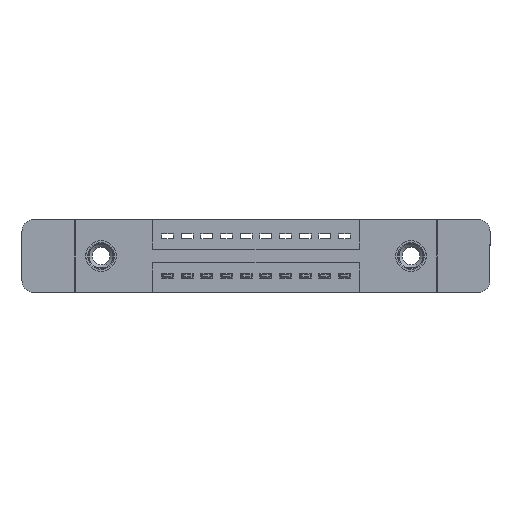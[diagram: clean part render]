
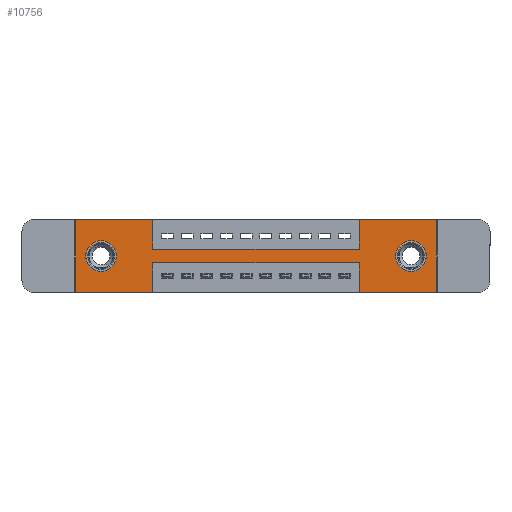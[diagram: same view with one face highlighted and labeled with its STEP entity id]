
A CAD part, front view. The second image highlights one B-rep face of the part: STEP entity #10756.
In plain terms, the highlighted planar face has unit normal (0, -1, 0).
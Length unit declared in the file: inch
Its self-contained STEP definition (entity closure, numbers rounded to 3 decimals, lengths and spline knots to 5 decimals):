
#69 = CARTESIAN_POINT ( 'NONE',  ( 0.3925, 0., -0.37 ) ) ;
#352 = VECTOR ( 'NONE', #3452, 39.37008 ) ;
#764 = VECTOR ( 'NONE', #14579, 39.37008 ) ;
#906 = LINE ( 'NONE', #8370, #14106 ) ;
#907 = ORIENTED_EDGE ( 'NONE', *, *, #7515, .T. ) ;
#1094 = DIRECTION ( 'NONE',  ( 1., 0., 0. ) ) ;
#1175 = VECTOR ( 'NONE', #15519, 39.37008 ) ;
#1199 = CARTESIAN_POINT ( 'NONE',  ( 0., 0., -0.37 ) ) ;
#1305 = DIRECTION ( 'NONE',  ( 1., 0., 0. ) ) ;
#1678 = DIRECTION ( 'NONE',  ( 0., 0., 1. ) ) ;
#1769 = LINE ( 'NONE', #69, #16605 ) ;
#1973 = EDGE_CURVE ( 'NONE', #7107, #16016, #13414, .T. ) ;
#2114 = FACE_OUTER_BOUND ( 'NONE', #6255, .T. ) ;
#2141 = VERTEX_POINT ( 'NONE', #15989 ) ;
#2217 = LINE ( 'NONE', #6424, #5238 ) ;
#2262 = ORIENTED_EDGE ( 'NONE', *, *, #8040, .F. ) ;
#2483 = DIRECTION ( 'NONE',  ( 0., -1., 0. ) ) ;
#2630 = VECTOR ( 'NONE', #10622, 39.37008 ) ;
#2729 = EDGE_CURVE ( 'NONE', #5162, #9375, #3029, .T. ) ;
#2741 = ORIENTED_EDGE ( 'NONE', *, *, #2940, .F. ) ;
#2897 = ORIENTED_EDGE ( 'NONE', *, *, #10849, .F. ) ;
#2940 = EDGE_CURVE ( 'NONE', #7504, #8922, #15925, .T. ) ;
#3029 = LINE ( 'NONE', #4997, #14016 ) ;
#3164 = CIRCLE ( 'NONE', #3179, 0.078 ) ;
#3179 = AXIS2_PLACEMENT_3D ( 'NONE', #3702, #4996, #6303 ) ;
#3452 = DIRECTION ( 'NONE',  ( -1., 0., 0. ) ) ;
#3506 = AXIS2_PLACEMENT_3D ( 'NONE', #15658, #6880, #13429 ) ;
#3511 = ORIENTED_EDGE ( 'NONE', *, *, #2729, .F. ) ;
#3568 = CARTESIAN_POINT ( 'NONE',  ( 1.4425, 0., 0. ) ) ;
#3702 = CARTESIAN_POINT ( 'NONE',  ( 1.705, 0., -0.185 ) ) ;
#3822 = DIRECTION ( 'NONE',  ( 1., 0., 0. ) ) ;
#3981 = CARTESIAN_POINT ( 'NONE',  ( 1.4425, 0., -0.22 ) ) ;
#4023 = CIRCLE ( 'NONE', #3506, 0.078 ) ;
#4073 = ORIENTED_EDGE ( 'NONE', *, *, #15768, .F. ) ;
#4182 = CARTESIAN_POINT ( 'NONE',  ( 0.3925, 0., 0. ) ) ;
#4228 = CARTESIAN_POINT ( 'NONE',  ( 0.13, 0., -0.107 ) ) ;
#4996 = DIRECTION ( 'NONE',  ( 0., 1., 0. ) ) ;
#4997 = CARTESIAN_POINT ( 'NONE',  ( 1.4425, 0., 0. ) ) ;
#5162 = VERTEX_POINT ( 'NONE', #7368 ) ;
#5234 = VERTEX_POINT ( 'NONE', #11166 ) ;
#5238 = VECTOR ( 'NONE', #11711, 39.37008 ) ;
#5241 = PLANE ( 'NONE',  #15727 ) ;
#5433 = VERTEX_POINT ( 'NONE', #11720 ) ;
#5545 = FACE_BOUND ( 'NONE', #5600, .T. ) ;
#5600 = EDGE_LOOP ( 'NONE', ( #14666, #7173 ) ) ;
#5824 = AXIS2_PLACEMENT_3D ( 'NONE', #11332, #7590, #7358 ) ;
#6061 = CIRCLE ( 'NONE', #14182, 0.078 ) ;
#6255 = EDGE_LOOP ( 'NONE', ( #2262, #4073, #2897, #14970, #8181, #15022, #3511, #14803, #2741, #13793, #12259, #10843 ) ) ;
#6303 = DIRECTION ( 'NONE',  ( 0., 0., -1. ) ) ;
#6424 = CARTESIAN_POINT ( 'NONE',  ( 0., 0., -0.37 ) ) ;
#6515 = CARTESIAN_POINT ( 'NONE',  ( 0.13, 0., -0.263 ) ) ;
#6685 = LINE ( 'NONE', #11953, #2630 ) ;
#6837 = EDGE_CURVE ( 'NONE', #2141, #7504, #12170, .T. ) ;
#6880 = DIRECTION ( 'NONE',  ( 0., 1., 0. ) ) ;
#6883 = DIRECTION ( 'NONE',  ( 0., 0., -1. ) ) ;
#6906 = EDGE_CURVE ( 'NONE', #7212, #5433, #2217, .T. ) ;
#7019 = LINE ( 'NONE', #11229, #352 ) ;
#7107 = VERTEX_POINT ( 'NONE', #11995 ) ;
#7173 = ORIENTED_EDGE ( 'NONE', *, *, #1973, .T. ) ;
#7212 = VERTEX_POINT ( 'NONE', #14894 ) ;
#7358 = DIRECTION ( 'NONE',  ( 0., 0., -1. ) ) ;
#7368 = CARTESIAN_POINT ( 'NONE',  ( 1.4425, 0., -0.15 ) ) ;
#7500 = ORIENTED_EDGE ( 'NONE', *, *, #12958, .T. ) ;
#7504 = VERTEX_POINT ( 'NONE', #12983 ) ;
#7515 = EDGE_CURVE ( 'NONE', #12425, #14979, #4023, .T. ) ;
#7590 = DIRECTION ( 'NONE',  ( 0., 1., 0. ) ) ;
#7779 = CARTESIAN_POINT ( 'NONE',  ( 1.4425, 0., -0.37 ) ) ;
#8040 = EDGE_CURVE ( 'NONE', #11811, #7212, #1769, .T. ) ;
#8067 = LINE ( 'NONE', #15754, #764 ) ;
#8181 = ORIENTED_EDGE ( 'NONE', *, *, #15499, .F. ) ;
#8287 = EDGE_CURVE ( 'NONE', #16415, #16197, #7019, .T. ) ;
#8370 = CARTESIAN_POINT ( 'NONE',  ( 1.4425, 0., -0.37 ) ) ;
#8707 = DIRECTION ( 'NONE',  ( 0., 0., 1. ) ) ;
#8922 = VERTEX_POINT ( 'NONE', #13014 ) ;
#9056 = VERTEX_POINT ( 'NONE', #3981 ) ;
#9169 = CARTESIAN_POINT ( 'NONE',  ( 0., 0., 0. ) ) ;
#9335 = DIRECTION ( 'NONE',  ( 0., 0., -1. ) ) ;
#9375 = VERTEX_POINT ( 'NONE', #3568 ) ;
#10256 = EDGE_LOOP ( 'NONE', ( #7500, #907 ) ) ;
#10622 = DIRECTION ( 'NONE',  ( 0., 0., 1. ) ) ;
#10756 = ADVANCED_FACE ( 'NONE', ( #5545, #11655, #2114 ), #5241, .T. ) ;
#10843 = ORIENTED_EDGE ( 'NONE', *, *, #6906, .F. ) ;
#10849 = EDGE_CURVE ( 'NONE', #16197, #9056, #906, .T. ) ;
#11002 = CARTESIAN_POINT ( 'NONE',  ( 1.705, 0., -0.107 ) ) ;
#11166 = CARTESIAN_POINT ( 'NONE',  ( 1.835, 0., 0. ) ) ;
#11229 = CARTESIAN_POINT ( 'NONE',  ( 0., 0., -0.37 ) ) ;
#11332 = CARTESIAN_POINT ( 'NONE',  ( 1.705, 0., -0.185 ) ) ;
#11397 = DIRECTION ( 'NONE',  ( 0., 1., 0. ) ) ;
#11622 = DIRECTION ( 'NONE',  ( 0., 0., 1. ) ) ;
#11655 = FACE_BOUND ( 'NONE', #10256, .T. ) ;
#11711 = DIRECTION ( 'NONE',  ( -1., 0., 0. ) ) ;
#11720 = CARTESIAN_POINT ( 'NONE',  ( 0., 0., -0.37 ) ) ;
#11811 = VERTEX_POINT ( 'NONE', #14137 ) ;
#11905 = VECTOR ( 'NONE', #1094, 39.37008 ) ;
#11953 = CARTESIAN_POINT ( 'NONE',  ( 0., 0., 0. ) ) ;
#11961 = CARTESIAN_POINT ( 'NONE',  ( 1.835, 0., -0.37 ) ) ;
#11995 = CARTESIAN_POINT ( 'NONE',  ( 1.705, 0., -0.263 ) ) ;
#12170 = LINE ( 'NONE', #14125, #14434 ) ;
#12259 = ORIENTED_EDGE ( 'NONE', *, *, #13176, .F. ) ;
#12425 = VERTEX_POINT ( 'NONE', #6515 ) ;
#12474 = VECTOR ( 'NONE', #6883, 39.37008 ) ;
#12883 = DIRECTION ( 'NONE',  ( 0., 0., -1. ) ) ;
#12958 = EDGE_CURVE ( 'NONE', #14979, #12425, #6061, .T. ) ;
#12983 = CARTESIAN_POINT ( 'NONE',  ( 0.3925, 0., 0. ) ) ;
#13014 = CARTESIAN_POINT ( 'NONE',  ( 0.3925, 0., -0.15 ) ) ;
#13176 = EDGE_CURVE ( 'NONE', #5433, #2141, #6685, .T. ) ;
#13414 = CIRCLE ( 'NONE', #5824, 0.078 ) ;
#13429 = DIRECTION ( 'NONE',  ( 0., 0., 1. ) ) ;
#13745 = LINE ( 'NONE', #9169, #16186 ) ;
#13793 = ORIENTED_EDGE ( 'NONE', *, *, #6837, .F. ) ;
#13996 = CARTESIAN_POINT ( 'NONE',  ( 0.3925, 0., -0.22 ) ) ;
#14016 = VECTOR ( 'NONE', #8707, 39.37008 ) ;
#14106 = VECTOR ( 'NONE', #1678, 39.37008 ) ;
#14125 = CARTESIAN_POINT ( 'NONE',  ( 0., 0., 0. ) ) ;
#14137 = CARTESIAN_POINT ( 'NONE',  ( 0.3925, 0., -0.22 ) ) ;
#14182 = AXIS2_PLACEMENT_3D ( 'NONE', #15486, #11397, #11622 ) ;
#14434 = VECTOR ( 'NONE', #3822, 39.37008 ) ;
#14579 = DIRECTION ( 'NONE',  ( 0., 0., -1. ) ) ;
#14666 = ORIENTED_EDGE ( 'NONE', *, *, #15824, .T. ) ;
#14768 = LINE ( 'NONE', #15340, #11905 ) ;
#14786 = EDGE_CURVE ( 'NONE', #9375, #5234, #13745, .T. ) ;
#14803 = ORIENTED_EDGE ( 'NONE', *, *, #16135, .F. ) ;
#14894 = CARTESIAN_POINT ( 'NONE',  ( 0.3925, 0., -0.37 ) ) ;
#14970 = ORIENTED_EDGE ( 'NONE', *, *, #8287, .F. ) ;
#14979 = VERTEX_POINT ( 'NONE', #4228 ) ;
#15022 = ORIENTED_EDGE ( 'NONE', *, *, #14786, .F. ) ;
#15340 = CARTESIAN_POINT ( 'NONE',  ( 0.3925, 0., -0.15 ) ) ;
#15486 = CARTESIAN_POINT ( 'NONE',  ( 0.13, 0., -0.185 ) ) ;
#15499 = EDGE_CURVE ( 'NONE', #5234, #16415, #8067, .T. ) ;
#15519 = DIRECTION ( 'NONE',  ( -1., 0., 0. ) ) ;
#15658 = CARTESIAN_POINT ( 'NONE',  ( 0.13, 0., -0.185 ) ) ;
#15727 = AXIS2_PLACEMENT_3D ( 'NONE', #1199, #2483, #12883 ) ;
#15754 = CARTESIAN_POINT ( 'NONE',  ( 1.835, 0., 0. ) ) ;
#15768 = EDGE_CURVE ( 'NONE', #9056, #11811, #15787, .T. ) ;
#15787 = LINE ( 'NONE', #13996, #1175 ) ;
#15824 = EDGE_CURVE ( 'NONE', #16016, #7107, #3164, .T. ) ;
#15925 = LINE ( 'NONE', #4182, #12474 ) ;
#15989 = CARTESIAN_POINT ( 'NONE',  ( 0., 0., 0. ) ) ;
#16016 = VERTEX_POINT ( 'NONE', #11002 ) ;
#16135 = EDGE_CURVE ( 'NONE', #8922, #5162, #14768, .T. ) ;
#16186 = VECTOR ( 'NONE', #1305, 39.37008 ) ;
#16197 = VERTEX_POINT ( 'NONE', #7779 ) ;
#16415 = VERTEX_POINT ( 'NONE', #11961 ) ;
#16605 = VECTOR ( 'NONE', #9335, 39.37008 ) ;
